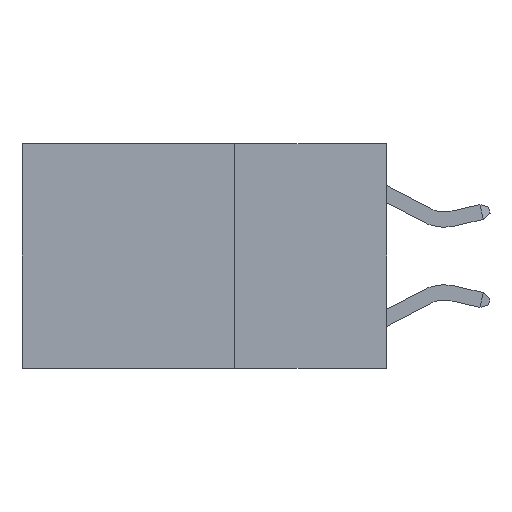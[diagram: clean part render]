
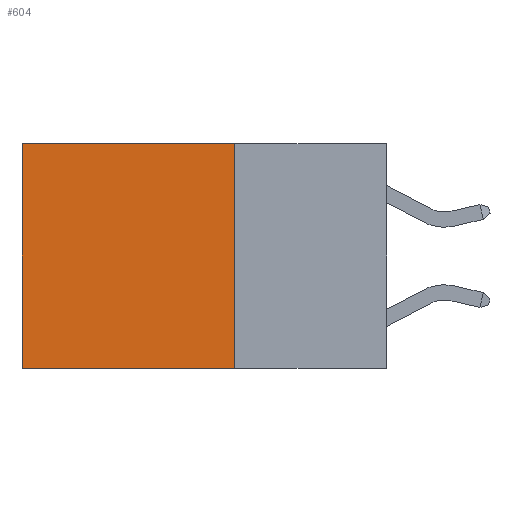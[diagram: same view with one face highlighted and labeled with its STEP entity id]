
A CAD part, left-side view. The second image highlights one B-rep face of the part: STEP entity #604.
In plain terms, the highlighted planar face has unit normal (-1, 0, 0).
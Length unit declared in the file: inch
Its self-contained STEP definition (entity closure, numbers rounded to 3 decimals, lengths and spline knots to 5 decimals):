
#62 = DIRECTION ( 'NONE',  ( 0., 1., 0. ) ) ;
#153 = DIRECTION ( 'NONE',  ( 0., 0., -1. ) ) ;
#604 = ADVANCED_FACE ( 'NONE', ( #26676 ), #26714, .F. ) ;
#2695 = LINE ( 'NONE', #5305, #27193 ) ;
#2869 = CARTESIAN_POINT ( 'NONE',  ( 0.2625, 0.25, 0. ) ) ;
#4335 = EDGE_LOOP ( 'NONE', ( #16422, #21946, #25317, #27991 ) ) ;
#5305 = CARTESIAN_POINT ( 'NONE',  ( 0.2625, 0.6, 0. ) ) ;
#6313 = AXIS2_PLACEMENT_3D ( 'NONE', #2869, #17189, #153 ) ;
#7697 = DIRECTION ( 'NONE',  ( 0., 0., -1. ) ) ;
#8241 = DIRECTION ( 'NONE',  ( 0., 0., -1. ) ) ;
#8541 = CARTESIAN_POINT ( 'NONE',  ( 0.2625, 0.25, -0.37 ) ) ;
#8769 = EDGE_CURVE ( 'NONE', #26778, #19469, #13651, .T. ) ;
#9206 = EDGE_CURVE ( 'NONE', #19469, #19395, #27127, .T. ) ;
#10469 = VECTOR ( 'NONE', #10925, 39.37008 ) ;
#10645 = CARTESIAN_POINT ( 'NONE',  ( 0.2625, 0.25, 0. ) ) ;
#10925 = DIRECTION ( 'NONE',  ( 0., 1., 0. ) ) ;
#12344 = VERTEX_POINT ( 'NONE', #13363 ) ;
#13307 = VECTOR ( 'NONE', #62, 39.37008 ) ;
#13363 = CARTESIAN_POINT ( 'NONE',  ( 0.2625, 0.6, 0. ) ) ;
#13651 = LINE ( 'NONE', #10645, #21093 ) ;
#15064 = EDGE_CURVE ( 'NONE', #12344, #19395, #2695, .T. ) ;
#15597 = EDGE_CURVE ( 'NONE', #26778, #12344, #25585, .T. ) ;
#16422 = ORIENTED_EDGE ( 'NONE', *, *, #15064, .T. ) ;
#17189 = DIRECTION ( 'NONE',  ( 1., 0., 0. ) ) ;
#19395 = VERTEX_POINT ( 'NONE', #20166 ) ;
#19469 = VERTEX_POINT ( 'NONE', #8541 ) ;
#20166 = CARTESIAN_POINT ( 'NONE',  ( 0.2625, 0.6, -0.37 ) ) ;
#21093 = VECTOR ( 'NONE', #8241, 39.37008 ) ;
#21946 = ORIENTED_EDGE ( 'NONE', *, *, #9206, .F. ) ;
#24790 = CARTESIAN_POINT ( 'NONE',  ( 0.2625, 0.25, 0. ) ) ;
#24909 = CARTESIAN_POINT ( 'NONE',  ( 0.2625, 0.25, -0.37 ) ) ;
#25317 = ORIENTED_EDGE ( 'NONE', *, *, #8769, .F. ) ;
#25585 = LINE ( 'NONE', #28731, #13307 ) ;
#26676 = FACE_OUTER_BOUND ( 'NONE', #4335, .T. ) ;
#26714 = PLANE ( 'NONE',  #6313 ) ;
#26778 = VERTEX_POINT ( 'NONE', #24790 ) ;
#27127 = LINE ( 'NONE', #24909, #10469 ) ;
#27193 = VECTOR ( 'NONE', #7697, 39.37008 ) ;
#27991 = ORIENTED_EDGE ( 'NONE', *, *, #15597, .T. ) ;
#28731 = CARTESIAN_POINT ( 'NONE',  ( 0.2625, 0.25, 0. ) ) ;
